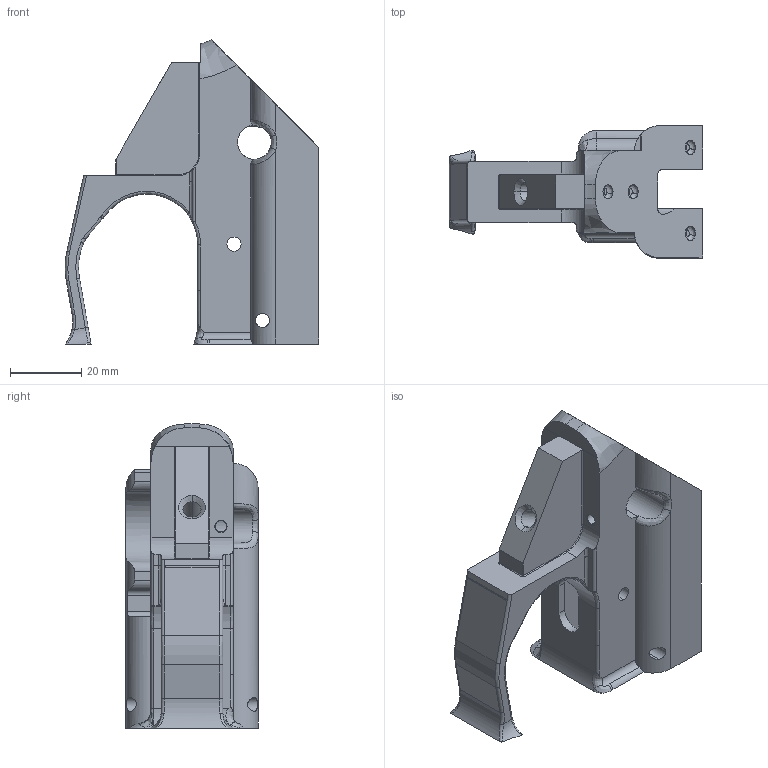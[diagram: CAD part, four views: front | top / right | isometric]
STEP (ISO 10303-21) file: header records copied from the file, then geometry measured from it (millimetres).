
FILE_DESCRIPTION (( 'STEP AP214' ), '1' );
FILE_NAME ('Vanilla_1.STEP', '2015-10-23T19:45:48', ( 'WarFairy' ), ( '' ), 'SwSTEP 2.0', 'SolidWorks 2015', '' );
FILE_SCHEMA (( 'AUTOMOTIVE_DESIGN' ));
Length unit declared in the file: millimetre
Products named in the file (1): Vanilla_1
Bounding box: 71.26 x 37.13 x 85.34 mm (x, y, z)
Volume: 49360.7 mm3; surface area: 20747.4 mm2
Topology: 1 solids, 1 shells, 211 faces, 576 edges, 365 vertices
Faces by surface type: cylinder 90, bspline 57, plane 48, torus 9, cone 4, sphere 3
Entity records: 16742 total; most frequent: CARTESIAN_POINT 11831, ORIENTED_EDGE 1128, DIRECTION 889, EDGE_CURVE 564, VERTEX_POINT 359, AXIS2_PLACEMENT_3D 333, EDGE_LOOP 233, VECTOR 223
